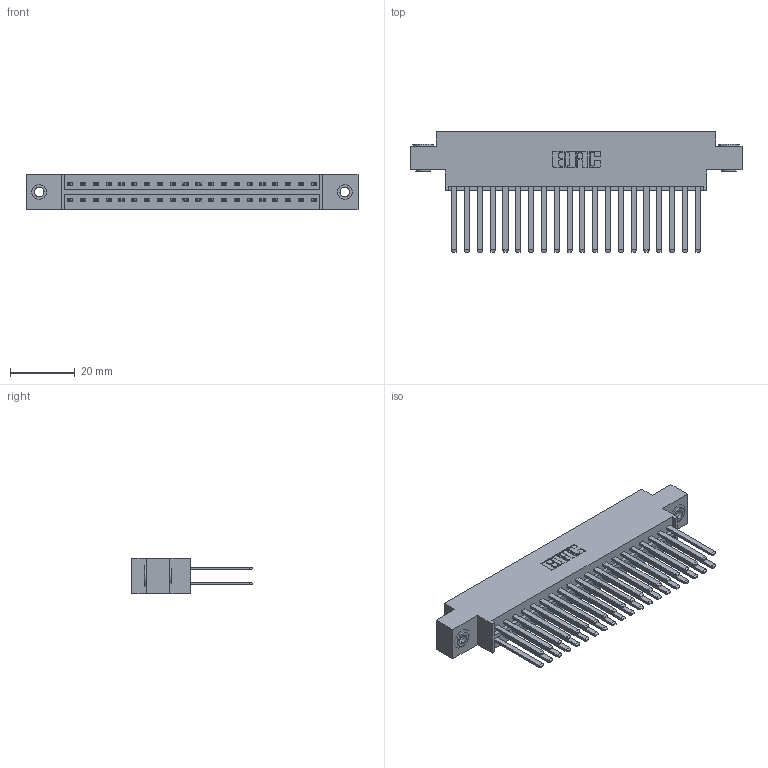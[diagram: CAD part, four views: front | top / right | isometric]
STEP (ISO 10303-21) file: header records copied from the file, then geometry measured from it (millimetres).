
FILE_DESCRIPTION (( 'STEP AP203' ), '1' );
FILE_NAME ('336-040-541-803.STEP', '2020-08-07T23:21:29', ( '' ), ( '' ), 'SwSTEP 2.0', 'SolidWorks 2020', '' );
FILE_SCHEMA (( 'CONFIG_CONTROL_DESIGN' ));
Length unit declared in the file: inch
Products named in the file (4): 336-040-541-803; 336-290-001_336-290-541; 336 Part_Offset - .156 Dia - TH; 345-250-002_345-250-002-102
Assembly tree (43 placements, depth 2):
  336-040-541-803
    336 Part_Offset - .156 Dia - TH
    336-290-001_336-290-541  x40
    345-250-002_345-250-002-102  x2
Bounding box: 102.64 x 37.34 x 11.1 mm (x, y, z)
Volume: 15149 mm3; surface area: 19218.7 mm2
Topology: 43 solids, 43 shells, 1836 faces, 5479 edges, 3622 vertices
Faces by surface type: plane 1124, cylinder 704, cone 8
Entity records: 18853 total; most frequent: CARTESIAN_POINT 3252, ORIENTED_EDGE 3082, DIRECTION 2743, EDGE_CURVE 1541, LINE 1385, VECTOR 1385, VERTEX_POINT 1024, AXIS2_PLACEMENT_3D 679
